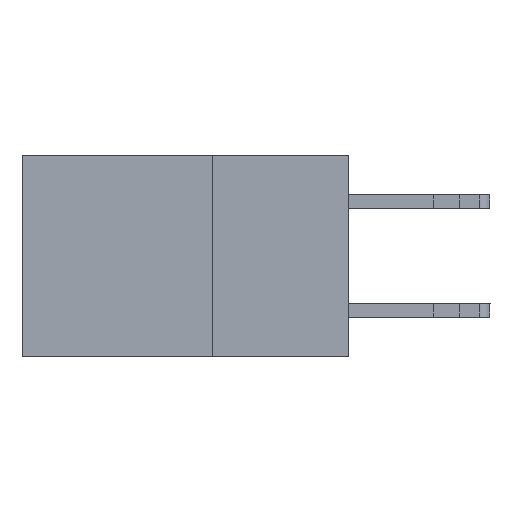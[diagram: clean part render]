
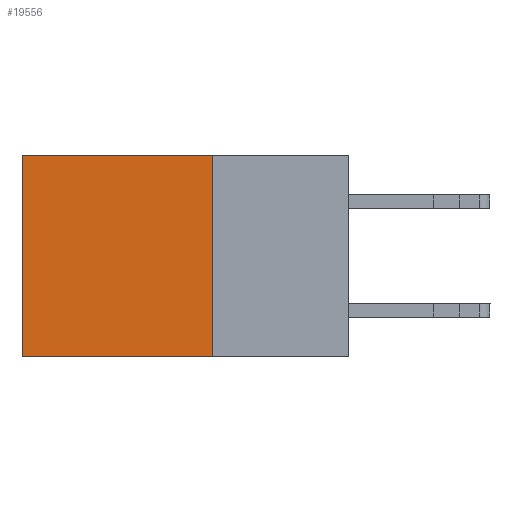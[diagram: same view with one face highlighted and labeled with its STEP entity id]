
A CAD part, left-side view. The second image highlights one B-rep face of the part: STEP entity #19556.
In plain terms, the highlighted planar face has unit normal (-1, 0, 0).
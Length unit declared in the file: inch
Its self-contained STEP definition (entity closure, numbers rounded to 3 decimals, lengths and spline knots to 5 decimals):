
#83 = DIRECTION ( 'NONE',  ( 0., 1., 0. ) ) ;
#1486 = LINE ( 'NONE', #8074, #3047 ) ;
#2244 = CARTESIAN_POINT ( 'NONE',  ( 0.298, 0.25, 0. ) ) ;
#2365 = AXIS2_PLACEMENT_3D ( 'NONE', #24628, #8448, #6760 ) ;
#2837 = DIRECTION ( 'NONE',  ( 0., 1., 0. ) ) ;
#3047 = VECTOR ( 'NONE', #83, 39.37008 ) ;
#3335 = FACE_OUTER_BOUND ( 'NONE', #24007, .T. ) ;
#3948 = CARTESIAN_POINT ( 'NONE',  ( 0.298, 0.6, 0. ) ) ;
#4187 = ORIENTED_EDGE ( 'NONE', *, *, #21272, .T. ) ;
#4662 = VECTOR ( 'NONE', #20124, 39.37008 ) ;
#5435 = CARTESIAN_POINT ( 'NONE',  ( 0.298, 0.6, -0.37 ) ) ;
#5896 = ORIENTED_EDGE ( 'NONE', *, *, #12675, .T. ) ;
#6760 = DIRECTION ( 'NONE',  ( 0., 0., -1. ) ) ;
#7295 = VERTEX_POINT ( 'NONE', #14563 ) ;
#7490 = LINE ( 'NONE', #2244, #4662 ) ;
#7842 = ORIENTED_EDGE ( 'NONE', *, *, #18394, .F. ) ;
#8065 = CARTESIAN_POINT ( 'NONE',  ( 0.298, 0.25, -0.37 ) ) ;
#8074 = CARTESIAN_POINT ( 'NONE',  ( 0.298, 0.25, 0. ) ) ;
#8448 = DIRECTION ( 'NONE',  ( 1., 0., 0. ) ) ;
#10594 = VERTEX_POINT ( 'NONE', #8065 ) ;
#12441 = CARTESIAN_POINT ( 'NONE',  ( 0.298, 0.25, -0.37 ) ) ;
#12640 = VERTEX_POINT ( 'NONE', #5435 ) ;
#12675 = EDGE_CURVE ( 'NONE', #17572, #7295, #1486, .T. ) ;
#13250 = VECTOR ( 'NONE', #2837, 39.37008 ) ;
#14255 = LINE ( 'NONE', #3948, #20010 ) ;
#14563 = CARTESIAN_POINT ( 'NONE',  ( 0.298, 0.6, 0. ) ) ;
#16442 = CARTESIAN_POINT ( 'NONE',  ( 0.298, 0.25, 0. ) ) ;
#16888 = EDGE_CURVE ( 'NONE', #10594, #12640, #23981, .T. ) ;
#17572 = VERTEX_POINT ( 'NONE', #16442 ) ;
#18016 = DIRECTION ( 'NONE',  ( 0., 0., -1. ) ) ;
#18152 = PLANE ( 'NONE',  #2365 ) ;
#18394 = EDGE_CURVE ( 'NONE', #17572, #10594, #7490, .T. ) ;
#19556 = ADVANCED_FACE ( 'NONE', ( #3335 ), #18152, .F. ) ;
#20010 = VECTOR ( 'NONE', #18016, 39.37008 ) ;
#20124 = DIRECTION ( 'NONE',  ( 0., 0., -1. ) ) ;
#21272 = EDGE_CURVE ( 'NONE', #7295, #12640, #14255, .T. ) ;
#21529 = ORIENTED_EDGE ( 'NONE', *, *, #16888, .F. ) ;
#23981 = LINE ( 'NONE', #12441, #13250 ) ;
#24007 = EDGE_LOOP ( 'NONE', ( #4187, #21529, #7842, #5896 ) ) ;
#24628 = CARTESIAN_POINT ( 'NONE',  ( 0.298, 0.25, 0. ) ) ;
